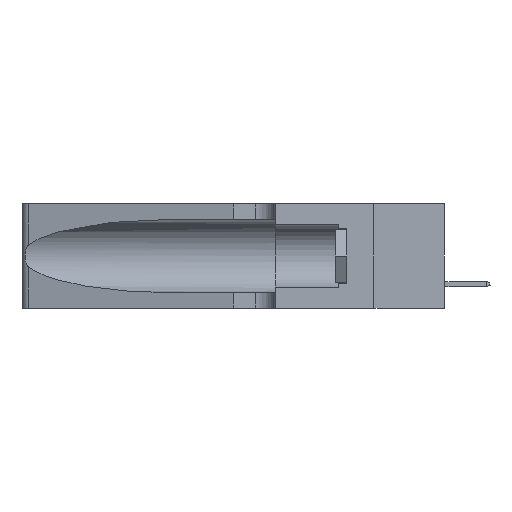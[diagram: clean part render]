
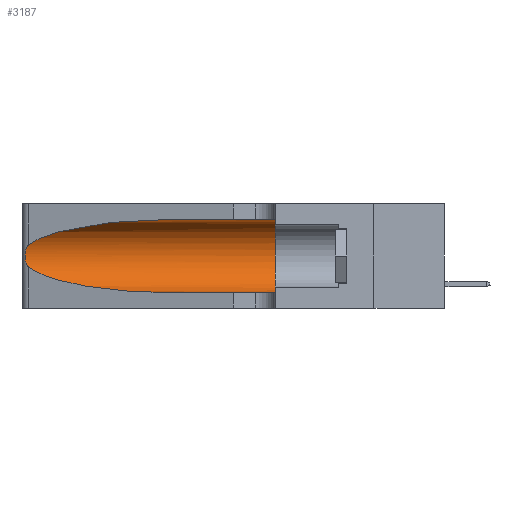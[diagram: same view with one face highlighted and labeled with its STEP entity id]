
A CAD part, left-side view. The second image highlights one B-rep face of the part: STEP entity #3187.
In plain terms, the highlighted cylindrical face has radius 3.308 mm (diameter 6.617 mm), a partial arc.
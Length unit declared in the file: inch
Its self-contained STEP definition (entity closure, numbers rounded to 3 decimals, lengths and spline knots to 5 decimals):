
#696 = CARTESIAN_POINT ( 'NONE',  ( 0.26075, 1.23896, 0.19203 ) ) ;
#1926 = ORIENTED_EDGE ( 'NONE', *, *, #13493, .T. ) ;
#2497 = DIRECTION ( 'NONE',  ( 0., 1., 0. ) ) ;
#3187 = ADVANCED_FACE ( 'NONE', ( #12284 ), #25305, .F. ) ;
#3440 = CARTESIAN_POINT ( 'NONE',  ( 0.1305, 0.72297, 0.31525 ) ) ;
#3546 = AXIS2_PLACEMENT_3D ( 'NONE', #6412, #2497, #8487 ) ;
#3953 = CARTESIAN_POINT ( 'NONE',  ( 0.25487, 1.22718, 0.14631 ) ) ;
#4084 = CARTESIAN_POINT ( 'NONE',  ( 0.1305, 1.61858, 0.185 ) ) ;
#4161 =( BOUNDED_CURVE ( )  B_SPLINE_CURVE ( 3, ( #25106, #10689, #4621, #24843 ),
 .UNSPECIFIED., .F., .F. ) 
 B_SPLINE_CURVE_WITH_KNOTS ( ( 4, 4 ),
 ( 3.44316, 4.71239 ),
 .UNSPECIFIED. ) 
 CURVE ( )  GEOMETRIC_REPRESENTATION_ITEM ( )  RATIONAL_B_SPLINE_CURVE ( ( 1., 0.87, 0.87, 1. ) ) 
 REPRESENTATION_ITEM ( '' )  );
#4550 = CARTESIAN_POINT ( 'NONE',  ( 0.25555, 1.22994, 0.2215 ) ) ;
#4621 = CARTESIAN_POINT ( 'NONE',  ( 0.18966, 0.96281, 0.05475 ) ) ;
#4635 = ORIENTED_EDGE ( 'NONE', *, *, #10139, .T. ) ;
#4811 = CARTESIAN_POINT ( 'NONE',  ( 0.26075, 1.23896, 0.178 ) ) ;
#4875 = LINE ( 'NONE', #15089, #7768 ) ;
#6113 = DIRECTION ( 'NONE',  ( 0., 0., -1. ) ) ;
#6296 = CARTESIAN_POINT ( 'NONE',  ( 0.1305, 1.61858, 0.31525 ) ) ;
#6412 = CARTESIAN_POINT ( 'NONE',  ( 0.1305, 0.35, 0.185 ) ) ;
#6559 = ORIENTED_EDGE ( 'NONE', *, *, #16567, .F. ) ;
#6781 = CARTESIAN_POINT ( 'NONE',  ( 0.25787, 1.23484, 0.2124 ) ) ;
#6866 = CARTESIAN_POINT ( 'NONE',  ( 0.26017, 1.23833, 0.17102 ) ) ;
#7534 = CARTESIAN_POINT ( 'NONE',  ( 0.2373, 1.15595, 0.28018 ) ) ;
#7768 = VECTOR ( 'NONE', #18901, 39.37008 ) ;
#7917 = CIRCLE ( 'NONE', #3546, 0.13025 ) ;
#8487 = DIRECTION ( 'NONE',  ( 0., 0., 1. ) ) ;
#8592 = CARTESIAN_POINT ( 'NONE',  ( 0.25856, 1.23593, 0.16098 ) ) ;
#8878 = EDGE_CURVE ( 'NONE', #21436, #19140, #19889, .T. ) ;
#9776 = CARTESIAN_POINT ( 'NONE',  ( 0.18966, 0.96281, 0.31525 ) ) ;
#10139 = EDGE_CURVE ( 'NONE', #17358, #11774, #4161, .T. ) ;
#10235 = DIRECTION ( 'NONE',  ( 0., -1., 0. ) ) ;
#10689 = CARTESIAN_POINT ( 'NONE',  ( 0.2373, 1.15595, 0.08982 ) ) ;
#10803 = CARTESIAN_POINT ( 'NONE',  ( 0.25639, 1.23184, 0.21858 ) ) ;
#11094 = VERTEX_POINT ( 'NONE', #12879 ) ;
#11239 = CARTESIAN_POINT ( 'NONE',  ( 0.1305, 0.72297, 0.05475 ) ) ;
#11774 = VERTEX_POINT ( 'NONE', #11239 ) ;
#11834 = CARTESIAN_POINT ( 'NONE',  ( 0.1305, 0.72297, 0.31525 ) ) ;
#11851 = EDGE_LOOP ( 'NONE', ( #11867, #24531, #4635, #1926, #6559, #18063 ) ) ;
#11867 = ORIENTED_EDGE ( 'NONE', *, *, #8878, .T. ) ;
#11926 = CARTESIAN_POINT ( 'NONE',  ( 0.25487, 1.22718, 0.22369 ) ) ;
#12284 = FACE_OUTER_BOUND ( 'NONE', #11851, .T. ) ;
#12850 = CARTESIAN_POINT ( 'NONE',  ( 0.25487, 1.22718, 0.14631 ) ) ;
#12879 = CARTESIAN_POINT ( 'NONE',  ( 0.1305, 0.35, 0.31525 ) ) ;
#13493 = EDGE_CURVE ( 'NONE', #11774, #23930, #4875, .T. ) ;
#15089 = CARTESIAN_POINT ( 'NONE',  ( 0.1305, 1.61858, 0.05475 ) ) ;
#16298 = EDGE_CURVE ( 'NONE', #19140, #17358, #17587, .T. ) ;
#16567 = EDGE_CURVE ( 'NONE', #11094, #23930, #7917, .T. ) ;
#17032 = CARTESIAN_POINT ( 'NONE',  ( 0.25854, 1.2359, 0.20912 ) ) ;
#17358 = VERTEX_POINT ( 'NONE', #3953 ) ;
#17526 = LINE ( 'NONE', #6296, #22327 ) ;
#17587 = B_SPLINE_CURVE_WITH_KNOTS ( 'NONE', 3,
 ( #20961, #4550, #10803, #6781, #17032, #20794, #696, #4811, #6866, #8592, #20885, #22930, #21151, #12850 ),
 .UNSPECIFIED., .F., .F.,
 ( 4, 2, 2, 2, 2, 2, 4 ),
 ( 0., 0.00027, 0.00053, 0.00107, 0.0016, 0.00187, 0.00214 ),
 .UNSPECIFIED. ) ;
#18063 = ORIENTED_EDGE ( 'NONE', *, *, #24404, .F. ) ;
#18901 = DIRECTION ( 'NONE',  ( 0., -1., 0. ) ) ;
#19140 = VERTEX_POINT ( 'NONE', #24805 ) ;
#19889 =( BOUNDED_CURVE ( )  B_SPLINE_CURVE ( 3, ( #3440, #9776, #7534, #11926 ),
 .UNSPECIFIED., .F., .F. ) 
 B_SPLINE_CURVE_WITH_KNOTS ( ( 4, 4 ),
 ( 1.5708, 2.84003 ),
 .UNSPECIFIED. ) 
 CURVE ( )  GEOMETRIC_REPRESENTATION_ITEM ( )  RATIONAL_B_SPLINE_CURVE ( ( 1., 0.87, 0.87, 1. ) ) 
 REPRESENTATION_ITEM ( '' )  );
#20055 = AXIS2_PLACEMENT_3D ( 'NONE', #4084, #10235, #6113 ) ;
#20794 = CARTESIAN_POINT ( 'NONE',  ( 0.26018, 1.23835, 0.19895 ) ) ;
#20885 = CARTESIAN_POINT ( 'NONE',  ( 0.25789, 1.23486, 0.15765 ) ) ;
#20961 = CARTESIAN_POINT ( 'NONE',  ( 0.25487, 1.22718, 0.22369 ) ) ;
#21039 = CARTESIAN_POINT ( 'NONE',  ( 0.1305, 0.35, 0.05475 ) ) ;
#21151 = CARTESIAN_POINT ( 'NONE',  ( 0.25555, 1.22993, 0.14849 ) ) ;
#21436 = VERTEX_POINT ( 'NONE', #11834 ) ;
#22327 = VECTOR ( 'NONE', #24673, 39.37008 ) ;
#22930 = CARTESIAN_POINT ( 'NONE',  ( 0.25639, 1.23186, 0.15144 ) ) ;
#23930 = VERTEX_POINT ( 'NONE', #21039 ) ;
#24404 = EDGE_CURVE ( 'NONE', #21436, #11094, #17526, .T. ) ;
#24531 = ORIENTED_EDGE ( 'NONE', *, *, #16298, .T. ) ;
#24673 = DIRECTION ( 'NONE',  ( 0., -1., 0. ) ) ;
#24805 = CARTESIAN_POINT ( 'NONE',  ( 0.25487, 1.22718, 0.22369 ) ) ;
#24843 = CARTESIAN_POINT ( 'NONE',  ( 0.1305, 0.72297, 0.05475 ) ) ;
#25106 = CARTESIAN_POINT ( 'NONE',  ( 0.25487, 1.22718, 0.14631 ) ) ;
#25305 = CYLINDRICAL_SURFACE ( 'NONE', #20055, 0.13025 ) ;
